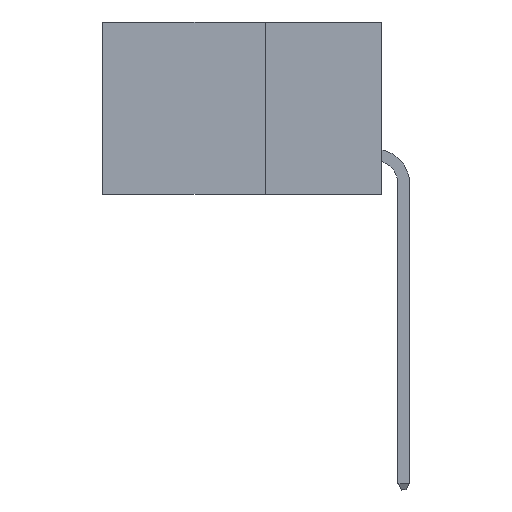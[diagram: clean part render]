
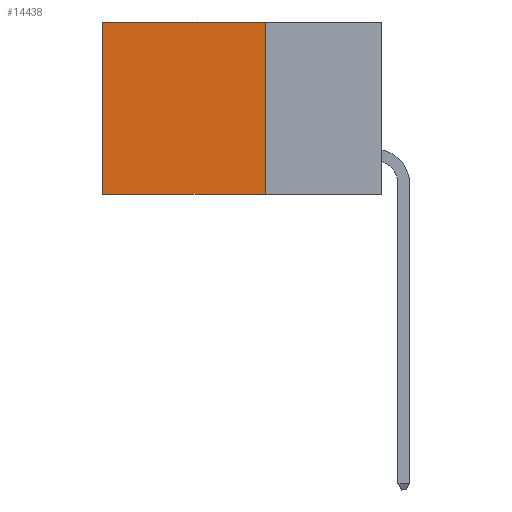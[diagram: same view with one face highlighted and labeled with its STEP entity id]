
A CAD part, left-side view. The second image highlights one B-rep face of the part: STEP entity #14438.
In plain terms, the highlighted planar face has unit normal (-1, 0, 0).
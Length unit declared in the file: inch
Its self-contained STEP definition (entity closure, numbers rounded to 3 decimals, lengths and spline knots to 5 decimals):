
#2097 = CARTESIAN_POINT ( 'NONE',  ( 0.2875, 0.25, 0. ) ) ;
#2228 = EDGE_CURVE ( 'NONE', #18954, #15226, #15326, .T. ) ;
#2379 = DIRECTION ( 'NONE',  ( 0., 0., -1. ) ) ;
#2463 = CARTESIAN_POINT ( 'NONE',  ( 0.2875, 0.6, 0. ) ) ;
#3124 = AXIS2_PLACEMENT_3D ( 'NONE', #3141, #22274, #20072 ) ;
#3141 = CARTESIAN_POINT ( 'NONE',  ( 0.2875, 0.25, 0. ) ) ;
#4848 = VECTOR ( 'NONE', #2379, 39.37008 ) ;
#4976 = PLANE ( 'NONE',  #3124 ) ;
#5189 = CARTESIAN_POINT ( 'NONE',  ( 0.2875, 0.6, -0.37 ) ) ;
#5387 = ORIENTED_EDGE ( 'NONE', *, *, #23685, .F. ) ;
#6186 = FACE_OUTER_BOUND ( 'NONE', #15190, .T. ) ;
#6519 = DIRECTION ( 'NONE',  ( 0., 0., -1. ) ) ;
#6707 = LINE ( 'NONE', #6786, #21714 ) ;
#6786 = CARTESIAN_POINT ( 'NONE',  ( 0.2875, 0.25, -0.37 ) ) ;
#6851 = ORIENTED_EDGE ( 'NONE', *, *, #19826, .T. ) ;
#8249 = LINE ( 'NONE', #10758, #17870 ) ;
#8698 = CARTESIAN_POINT ( 'NONE',  ( 0.2875, 0.6, 0. ) ) ;
#8920 = CARTESIAN_POINT ( 'NONE',  ( 0.2875, 0.25, -0.37 ) ) ;
#9521 = LINE ( 'NONE', #16047, #10127 ) ;
#10127 = VECTOR ( 'NONE', #6519, 39.37008 ) ;
#10758 = CARTESIAN_POINT ( 'NONE',  ( 0.2875, 0.25, 0. ) ) ;
#13441 = VERTEX_POINT ( 'NONE', #2097 ) ;
#14438 = ADVANCED_FACE ( 'NONE', ( #6186 ), #4976, .F. ) ;
#15003 = ORIENTED_EDGE ( 'NONE', *, *, #2228, .T. ) ;
#15190 = EDGE_LOOP ( 'NONE', ( #15003, #15895, #5387, #6851 ) ) ;
#15226 = VERTEX_POINT ( 'NONE', #5189 ) ;
#15326 = LINE ( 'NONE', #2463, #4848 ) ;
#15895 = ORIENTED_EDGE ( 'NONE', *, *, #16398, .F. ) ;
#16047 = CARTESIAN_POINT ( 'NONE',  ( 0.2875, 0.25, 0. ) ) ;
#16398 = EDGE_CURVE ( 'NONE', #17167, #15226, #6707, .T. ) ;
#17167 = VERTEX_POINT ( 'NONE', #8920 ) ;
#17870 = VECTOR ( 'NONE', #18638, 39.37008 ) ;
#18356 = DIRECTION ( 'NONE',  ( 0., 1., 0. ) ) ;
#18638 = DIRECTION ( 'NONE',  ( 0., 1., 0. ) ) ;
#18954 = VERTEX_POINT ( 'NONE', #8698 ) ;
#19826 = EDGE_CURVE ( 'NONE', #13441, #18954, #8249, .T. ) ;
#20072 = DIRECTION ( 'NONE',  ( 0., 0., -1. ) ) ;
#21714 = VECTOR ( 'NONE', #18356, 39.37008 ) ;
#22274 = DIRECTION ( 'NONE',  ( 1., 0., 0. ) ) ;
#23685 = EDGE_CURVE ( 'NONE', #13441, #17167, #9521, .T. ) ;
